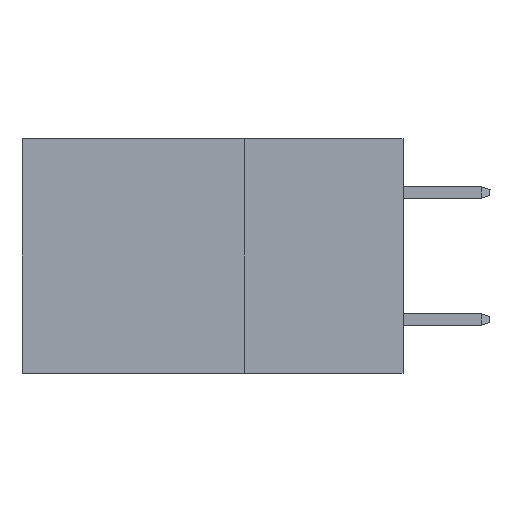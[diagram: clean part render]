
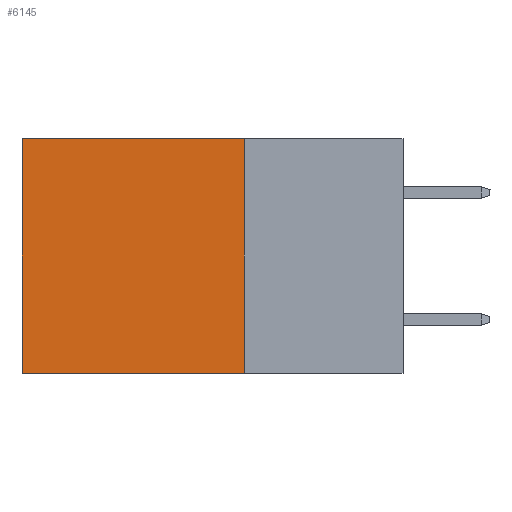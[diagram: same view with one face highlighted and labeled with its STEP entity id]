
A CAD part, left-side view. The second image highlights one B-rep face of the part: STEP entity #6145.
In plain terms, the highlighted planar face has unit normal (-1, 0, 0).
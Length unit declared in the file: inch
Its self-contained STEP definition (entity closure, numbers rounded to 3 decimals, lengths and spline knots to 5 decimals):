
#314 = PLANE ( 'NONE',  #6370 ) ;
#369 = VECTOR ( 'NONE', #2875, 39.37008 ) ;
#438 = CARTESIAN_POINT ( 'NONE',  ( 0.2875, 0.25, 0. ) ) ;
#789 = ORIENTED_EDGE ( 'NONE', *, *, #10092, .F. ) ;
#1362 = CARTESIAN_POINT ( 'NONE',  ( 0.2875, 0.6, 0. ) ) ;
#1604 = DIRECTION ( 'NONE',  ( 0., 1., 0. ) ) ;
#2004 = VERTEX_POINT ( 'NONE', #6386 ) ;
#2257 = VECTOR ( 'NONE', #1604, 39.37008 ) ;
#2280 = FACE_OUTER_BOUND ( 'NONE', #9575, .T. ) ;
#2607 = CARTESIAN_POINT ( 'NONE',  ( 0.2875, 0.6, 0. ) ) ;
#2785 = VERTEX_POINT ( 'NONE', #8362 ) ;
#2875 = DIRECTION ( 'NONE',  ( 0., 0., -1. ) ) ;
#2928 = ORIENTED_EDGE ( 'NONE', *, *, #8188, .F. ) ;
#3325 = DIRECTION ( 'NONE',  ( 0., 0., -1. ) ) ;
#4646 = LINE ( 'NONE', #9627, #8667 ) ;
#4669 = EDGE_CURVE ( 'NONE', #10561, #2785, #12577, .T. ) ;
#5046 = CARTESIAN_POINT ( 'NONE',  ( 0.2875, 0.25, 0. ) ) ;
#5156 = LINE ( 'NONE', #5046, #8280 ) ;
#5660 = ORIENTED_EDGE ( 'NONE', *, *, #4669, .T. ) ;
#6079 = ORIENTED_EDGE ( 'NONE', *, *, #10659, .T. ) ;
#6145 = ADVANCED_FACE ( 'NONE', ( #2280 ), #314, .F. ) ;
#6234 = DIRECTION ( 'NONE',  ( 1., 0., 0. ) ) ;
#6370 = AXIS2_PLACEMENT_3D ( 'NONE', #438, #6234, #3325 ) ;
#6386 = CARTESIAN_POINT ( 'NONE',  ( 0.2875, 0.25, 0. ) ) ;
#7269 = CARTESIAN_POINT ( 'NONE',  ( 0.2875, 0.25, 0. ) ) ;
#7462 = VERTEX_POINT ( 'NONE', #7978 ) ;
#7757 = DIRECTION ( 'NONE',  ( 0., 1., 0. ) ) ;
#7978 = CARTESIAN_POINT ( 'NONE',  ( 0.2875, 0.25, -0.37 ) ) ;
#8188 = EDGE_CURVE ( 'NONE', #2004, #7462, #5156, .T. ) ;
#8280 = VECTOR ( 'NONE', #9105, 39.37008 ) ;
#8362 = CARTESIAN_POINT ( 'NONE',  ( 0.2875, 0.6, -0.37 ) ) ;
#8667 = VECTOR ( 'NONE', #7757, 39.37008 ) ;
#9105 = DIRECTION ( 'NONE',  ( 0., 0., -1. ) ) ;
#9575 = EDGE_LOOP ( 'NONE', ( #5660, #789, #2928, #6079 ) ) ;
#9627 = CARTESIAN_POINT ( 'NONE',  ( 0.2875, 0.25, -0.37 ) ) ;
#10092 = EDGE_CURVE ( 'NONE', #7462, #2785, #4646, .T. ) ;
#10461 = LINE ( 'NONE', #7269, #2257 ) ;
#10561 = VERTEX_POINT ( 'NONE', #1362 ) ;
#10659 = EDGE_CURVE ( 'NONE', #2004, #10561, #10461, .T. ) ;
#12577 = LINE ( 'NONE', #2607, #369 ) ;
